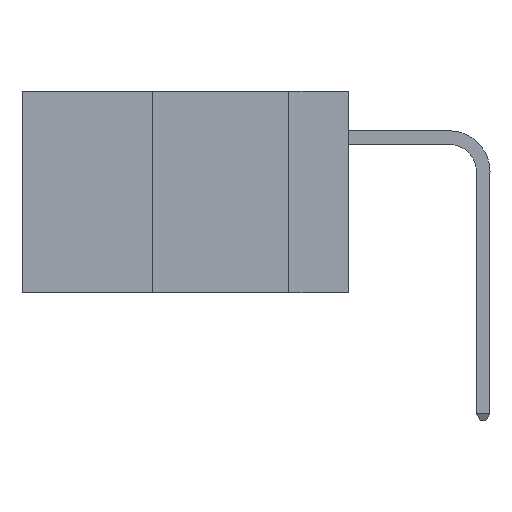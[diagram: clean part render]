
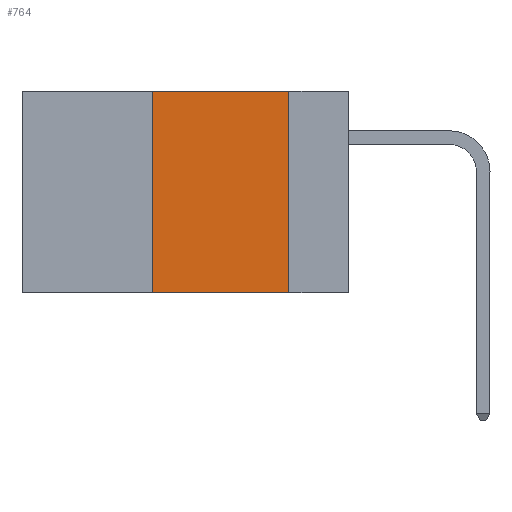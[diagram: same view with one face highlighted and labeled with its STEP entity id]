
A CAD part, left-side view. The second image highlights one B-rep face of the part: STEP entity #764.
In plain terms, the highlighted planar face has unit normal (-1, 0, 0).
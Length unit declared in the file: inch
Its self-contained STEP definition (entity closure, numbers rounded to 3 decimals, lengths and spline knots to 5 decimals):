
#642 = DIRECTION ( 'NONE',  ( 0., 0., 1. ) ) ;
#764 = ADVANCED_FACE ( 'NONE', ( #20291 ), #11822, .F. ) ;
#895 = DIRECTION ( 'NONE',  ( 0., -1., 0. ) ) ;
#967 = VECTOR ( 'NONE', #21422, 39.37008 ) ;
#1002 = LINE ( 'NONE', #19218, #1541 ) ;
#1541 = VECTOR ( 'NONE', #642, 39.37008 ) ;
#1564 = LINE ( 'NONE', #19976, #2092 ) ;
#2092 = VECTOR ( 'NONE', #10062, 39.37008 ) ;
#2941 = CARTESIAN_POINT ( 'NONE',  ( 0., 0.6, -0.37 ) ) ;
#2975 = CARTESIAN_POINT ( 'NONE',  ( 0., 0.36, 0. ) ) ;
#3116 = ORIENTED_EDGE ( 'NONE', *, *, #6312, .F. ) ;
#4321 = EDGE_CURVE ( 'NONE', #18929, #10658, #14652, .T. ) ;
#4900 = EDGE_LOOP ( 'NONE', ( #14363, #15632, #3116, #7750 ) ) ;
#5003 = DIRECTION ( 'NONE',  ( 0., 0., -1. ) ) ;
#5174 = EDGE_CURVE ( 'NONE', #10658, #6002, #1564, .T. ) ;
#6002 = VERTEX_POINT ( 'NONE', #8130 ) ;
#6312 = EDGE_CURVE ( 'NONE', #13910, #18929, #1002, .T. ) ;
#7612 = AXIS2_PLACEMENT_3D ( 'NONE', #13486, #15162, #5003 ) ;
#7750 = ORIENTED_EDGE ( 'NONE', *, *, #13161, .T. ) ;
#8130 = CARTESIAN_POINT ( 'NONE',  ( 0., 0.11, -0.37 ) ) ;
#8378 = CARTESIAN_POINT ( 'NONE',  ( 0., 0.36, -0.37 ) ) ;
#9308 = CARTESIAN_POINT ( 'NONE',  ( 0., 0.11, 0. ) ) ;
#10062 = DIRECTION ( 'NONE',  ( 0., 0., -1. ) ) ;
#10136 = LINE ( 'NONE', #2941, #967 ) ;
#10658 = VERTEX_POINT ( 'NONE', #9308 ) ;
#11822 = PLANE ( 'NONE',  #7612 ) ;
#13161 = EDGE_CURVE ( 'NONE', #13910, #6002, #10136, .T. ) ;
#13486 = CARTESIAN_POINT ( 'NONE',  ( 0., 0.6, 0. ) ) ;
#13910 = VERTEX_POINT ( 'NONE', #8378 ) ;
#14363 = ORIENTED_EDGE ( 'NONE', *, *, #5174, .F. ) ;
#14652 = LINE ( 'NONE', #17847, #19059 ) ;
#15162 = DIRECTION ( 'NONE',  ( 1., 0., 0. ) ) ;
#15632 = ORIENTED_EDGE ( 'NONE', *, *, #4321, .F. ) ;
#17847 = CARTESIAN_POINT ( 'NONE',  ( 0., 0.6, 0. ) ) ;
#18929 = VERTEX_POINT ( 'NONE', #2975 ) ;
#19059 = VECTOR ( 'NONE', #895, 39.37008 ) ;
#19218 = CARTESIAN_POINT ( 'NONE',  ( 0., 0.36, 0. ) ) ;
#19976 = CARTESIAN_POINT ( 'NONE',  ( 0., 0.11, 0. ) ) ;
#20291 = FACE_OUTER_BOUND ( 'NONE', #4900, .T. ) ;
#21422 = DIRECTION ( 'NONE',  ( 0., -1., 0. ) ) ;
